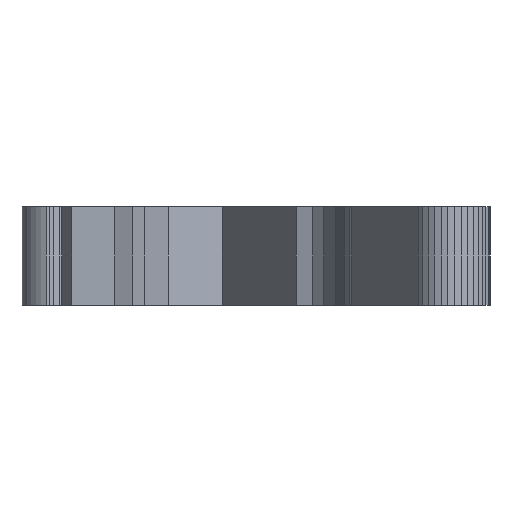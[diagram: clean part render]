
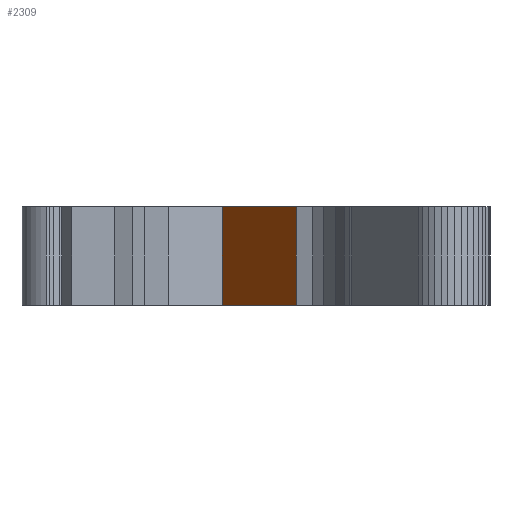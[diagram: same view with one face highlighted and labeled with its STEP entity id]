
A CAD part, front view. The second image highlights one B-rep face of the part: STEP entity #2309.
In plain terms, the highlighted planar face has unit normal (-0.832, -0.554, 0).
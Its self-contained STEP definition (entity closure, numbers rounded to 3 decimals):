
#2253=CARTESIAN_POINT('',(-13.314,9.635,0.0));
#2254=VERTEX_POINT('',#2253);
#2262=CARTESIAN_POINT('',(-13.314,9.635,11.0));
#2263=VERTEX_POINT('',#2262);
#2270=CARTESIAN_POINT('',(-13.314,9.635,0.0));
#2271=DIRECTION('',(0.0,0.0,1.0));
#2272=VECTOR('',#2271,11.0);
#2273=LINE('',#2270,#2272);
#2274=EDGE_CURVE('',#2254,#2263,#2273,.T.);
#2279=CARTESIAN_POINT('',(-21.61,22.094,0.0));
#2280=DIRECTION('',(-0.832,-0.554,0.0));
#2281=DIRECTION('',(0.554,-0.832,0.0));
#2282=AXIS2_PLACEMENT_3D('',#2279,#2280,#2281);
#2283=PLANE('',#2282);
#2284=CARTESIAN_POINT('',(-21.61,22.094,0.0));
#2285=VERTEX_POINT('',#2284);
#2286=CARTESIAN_POINT('',(-21.61,22.094,0.0));
#2287=DIRECTION('',(0.554,-0.832,0.0));
#2288=VECTOR('',#2287,14.968);
#2289=LINE('',#2286,#2288);
#2290=EDGE_CURVE('',#2285,#2254,#2289,.T.);
#2291=ORIENTED_EDGE('',*,*,#2290,.T.);
#2292=ORIENTED_EDGE('',*,*,#2274,.T.);
#2293=CARTESIAN_POINT('',(-21.61,22.094,11.0));
#2294=VERTEX_POINT('',#2293);
#2295=CARTESIAN_POINT('',(-21.61,22.094,11.0));
#2296=DIRECTION('',(0.554,-0.832,0.0));
#2297=VECTOR('',#2296,14.968);
#2298=LINE('',#2295,#2297);
#2299=EDGE_CURVE('',#2294,#2263,#2298,.T.);
#2300=ORIENTED_EDGE('',*,*,#2299,.F.);
#2301=CARTESIAN_POINT('',(-21.61,22.094,0.0));
#2302=DIRECTION('',(0.0,0.0,1.0));
#2303=VECTOR('',#2302,11.0);
#2304=LINE('',#2301,#2303);
#2305=EDGE_CURVE('',#2285,#2294,#2304,.T.);
#2306=ORIENTED_EDGE('',*,*,#2305,.F.);
#2307=EDGE_LOOP('',(#2291,#2292,#2300,#2306));
#2308=FACE_OUTER_BOUND('',#2307,.T.);
#2309=ADVANCED_FACE('',(#2308),#2283,.T.);
